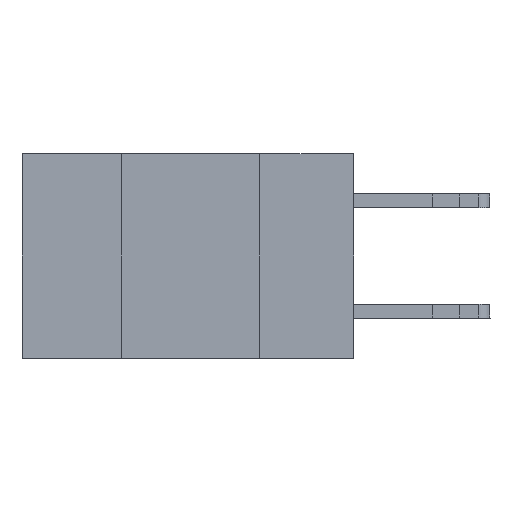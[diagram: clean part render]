
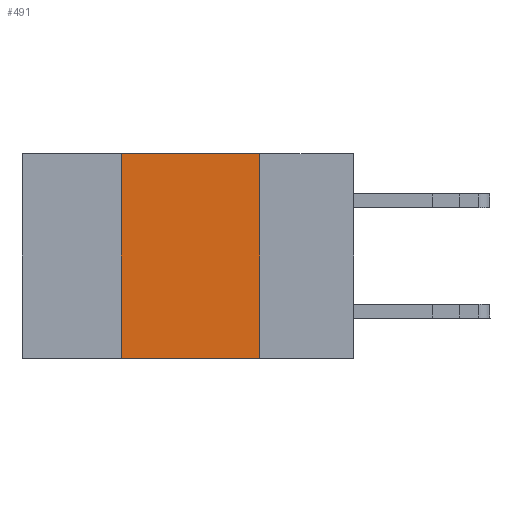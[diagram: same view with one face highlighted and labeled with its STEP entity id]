
A CAD part, left-side view. The second image highlights one B-rep face of the part: STEP entity #491.
In plain terms, the highlighted planar face has unit normal (-1, 0, 0).
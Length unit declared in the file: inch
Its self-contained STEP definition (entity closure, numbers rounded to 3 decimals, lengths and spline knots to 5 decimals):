
#128 = DIRECTION ( 'NONE',  ( 0., -1., 0. ) ) ;
#368 = CARTESIAN_POINT ( 'NONE',  ( 0., 0.6, -0.37 ) ) ;
#491 = ADVANCED_FACE ( 'NONE', ( #5624 ), #11267, .F. ) ;
#830 = CARTESIAN_POINT ( 'NONE',  ( 0., 0.17, 0. ) ) ;
#1160 = DIRECTION ( 'NONE',  ( 0., 0., -1. ) ) ;
#1724 = LINE ( 'NONE', #25181, #20134 ) ;
#2904 = CARTESIAN_POINT ( 'NONE',  ( 0., 0.42, -0.37 ) ) ;
#5624 = FACE_OUTER_BOUND ( 'NONE', #24592, .T. ) ;
#8048 = DIRECTION ( 'NONE',  ( 0., -1., 0. ) ) ;
#8375 = LINE ( 'NONE', #368, #10255 ) ;
#9851 = DIRECTION ( 'NONE',  ( 1., 0., 0. ) ) ;
#10075 = VERTEX_POINT ( 'NONE', #16950 ) ;
#10255 = VECTOR ( 'NONE', #8048, 39.37008 ) ;
#11204 = VERTEX_POINT ( 'NONE', #830 ) ;
#11267 = PLANE ( 'NONE',  #15031 ) ;
#11496 = ORIENTED_EDGE ( 'NONE', *, *, #21548, .F. ) ;
#11764 = VECTOR ( 'NONE', #128, 39.37008 ) ;
#13013 = VERTEX_POINT ( 'NONE', #2904 ) ;
#13246 = DIRECTION ( 'NONE',  ( 0., 0., -1. ) ) ;
#13323 = ORIENTED_EDGE ( 'NONE', *, *, #18983, .F. ) ;
#13425 = CARTESIAN_POINT ( 'NONE',  ( 0., 0.6, 0. ) ) ;
#14855 = ORIENTED_EDGE ( 'NONE', *, *, #17085, .F. ) ;
#15031 = AXIS2_PLACEMENT_3D ( 'NONE', #13425, #9851, #13246 ) ;
#15855 = CARTESIAN_POINT ( 'NONE',  ( 0., 0.6, 0. ) ) ;
#16053 = EDGE_CURVE ( 'NONE', #13013, #23074, #8375, .T. ) ;
#16950 = CARTESIAN_POINT ( 'NONE',  ( 0., 0.42, 0. ) ) ;
#17082 = LINE ( 'NONE', #15855, #11764 ) ;
#17085 = EDGE_CURVE ( 'NONE', #10075, #11204, #17082, .T. ) ;
#18983 = EDGE_CURVE ( 'NONE', #11204, #23074, #1724, .T. ) ;
#19462 = VECTOR ( 'NONE', #20216, 39.37008 ) ;
#19526 = CARTESIAN_POINT ( 'NONE',  ( 0., 0.17, -0.37 ) ) ;
#20134 = VECTOR ( 'NONE', #1160, 39.37008 ) ;
#20216 = DIRECTION ( 'NONE',  ( 0., 0., 1. ) ) ;
#20569 = CARTESIAN_POINT ( 'NONE',  ( 0., 0.42, 0. ) ) ;
#21342 = LINE ( 'NONE', #20569, #19462 ) ;
#21548 = EDGE_CURVE ( 'NONE', #13013, #10075, #21342, .T. ) ;
#23074 = VERTEX_POINT ( 'NONE', #19526 ) ;
#24592 = EDGE_LOOP ( 'NONE', ( #13323, #14855, #11496, #24799 ) ) ;
#24799 = ORIENTED_EDGE ( 'NONE', *, *, #16053, .T. ) ;
#25181 = CARTESIAN_POINT ( 'NONE',  ( 0., 0.17, 0. ) ) ;
